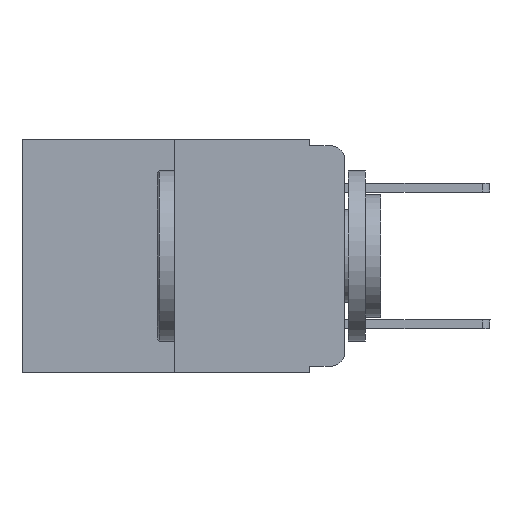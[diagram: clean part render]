
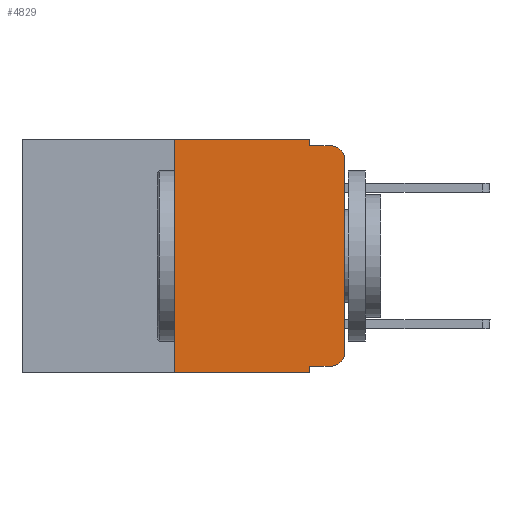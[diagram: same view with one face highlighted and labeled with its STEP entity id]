
A CAD part, left-side view. The second image highlights one B-rep face of the part: STEP entity #4829.
In plain terms, the highlighted planar face has unit normal (-1, 0, 0).
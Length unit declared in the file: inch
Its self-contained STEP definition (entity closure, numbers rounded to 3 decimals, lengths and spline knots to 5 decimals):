
#119 = CARTESIAN_POINT ( 'NONE',  ( 0., 0.25, 0. ) ) ;
#269 = DIRECTION ( 'NONE',  ( 0., 0., 1. ) ) ;
#2017 = ORIENTED_EDGE ( 'NONE', *, *, #8994, .T. ) ;
#2059 = CARTESIAN_POINT ( 'NONE',  ( 0., 0.051, 0. ) ) ;
#2314 = DIRECTION ( 'NONE',  ( 0., 0., -1. ) ) ;
#2352 = LINE ( 'NONE', #2059, #9926 ) ;
#2513 = CARTESIAN_POINT ( 'NONE',  ( 0., 0.051, 0. ) ) ;
#2537 = VECTOR ( 'NONE', #18126, 39.37008 ) ;
#2985 = ORIENTED_EDGE ( 'NONE', *, *, #7455, .T. ) ;
#3214 = VERTEX_POINT ( 'NONE', #12485 ) ;
#3493 = CARTESIAN_POINT ( 'NONE',  ( 0., 0.473, 0. ) ) ;
#3868 = ORIENTED_EDGE ( 'NONE', *, *, #16615, .T. ) ;
#4252 = CARTESIAN_POINT ( 'NONE',  ( 0., 0.051, -0.333 ) ) ;
#4829 = ADVANCED_FACE ( 'NONE', ( #7254 ), #5104, .F. ) ;
#5104 = PLANE ( 'NONE',  #19816 ) ;
#5206 = CARTESIAN_POINT ( 'NONE',  ( 0., 0.02, -0.01 ) ) ;
#5267 = CARTESIAN_POINT ( 'NONE',  ( 0., 0.051, -0.343 ) ) ;
#5402 = ORIENTED_EDGE ( 'NONE', *, *, #12630, .F. ) ;
#5836 = CIRCLE ( 'NONE', #9157, 0.02 ) ;
#5852 = ORIENTED_EDGE ( 'NONE', *, *, #18767, .F. ) ;
#6549 = EDGE_CURVE ( 'NONE', #10947, #18829, #18730, .T. ) ;
#6596 = CARTESIAN_POINT ( 'NONE',  ( 0., 0.473, 0. ) ) ;
#6755 = CARTESIAN_POINT ( 'NONE',  ( 0., 0.25, 0. ) ) ;
#6917 = VECTOR ( 'NONE', #20727, 39.37008 ) ;
#7033 = DIRECTION ( 'NONE',  ( 0., 0., -1. ) ) ;
#7208 = VERTEX_POINT ( 'NONE', #19360 ) ;
#7254 = FACE_OUTER_BOUND ( 'NONE', #12192, .T. ) ;
#7363 = LINE ( 'NONE', #6755, #19156 ) ;
#7409 = CARTESIAN_POINT ( 'NONE',  ( 0., 0., -0.03 ) ) ;
#7455 = EDGE_CURVE ( 'NONE', #20374, #13976, #18947, .T. ) ;
#7466 = ORIENTED_EDGE ( 'NONE', *, *, #17166, .T. ) ;
#7509 = CARTESIAN_POINT ( 'NONE',  ( 0., 0., 0. ) ) ;
#7764 = ORIENTED_EDGE ( 'NONE', *, *, #14862, .T. ) ;
#7814 = VERTEX_POINT ( 'NONE', #18473 ) ;
#8141 = CARTESIAN_POINT ( 'NONE',  ( 0., 0.051, 0. ) ) ;
#8751 = LINE ( 'NONE', #3493, #16274 ) ;
#8805 = CARTESIAN_POINT ( 'NONE',  ( 0., 0.02, -0.03 ) ) ;
#8957 = DIRECTION ( 'NONE',  ( 0., 0., 1. ) ) ;
#8964 = EDGE_CURVE ( 'NONE', #7208, #14667, #7363, .T. ) ;
#8994 = EDGE_CURVE ( 'NONE', #20361, #7814, #5836, .T. ) ;
#9001 = EDGE_CURVE ( 'NONE', #17385, #3214, #2352, .T. ) ;
#9157 = AXIS2_PLACEMENT_3D ( 'NONE', #10116, #10189, #7033 ) ;
#9716 = LINE ( 'NONE', #4252, #6917 ) ;
#9736 = VECTOR ( 'NONE', #13779, 39.37008 ) ;
#9838 = ORIENTED_EDGE ( 'NONE', *, *, #8964, .F. ) ;
#9926 = VECTOR ( 'NONE', #11877, 39.37008 ) ;
#10116 = CARTESIAN_POINT ( 'NONE',  ( 0., 0.02, -0.313 ) ) ;
#10189 = DIRECTION ( 'NONE',  ( -1., 0., 0. ) ) ;
#10475 = VECTOR ( 'NONE', #14422, 39.37008 ) ;
#10500 = CARTESIAN_POINT ( 'NONE',  ( 0., 0.02, -0.333 ) ) ;
#10947 = VERTEX_POINT ( 'NONE', #12155 ) ;
#11160 = ORIENTED_EDGE ( 'NONE', *, *, #6549, .F. ) ;
#11381 = DIRECTION ( 'NONE',  ( 1., 0., 0. ) ) ;
#11719 = DIRECTION ( 'NONE',  ( -1., 0., 0. ) ) ;
#11877 = DIRECTION ( 'NONE',  ( 0., 0., -1. ) ) ;
#12155 = CARTESIAN_POINT ( 'NONE',  ( 0., 0.051, -0.333 ) ) ;
#12192 = EDGE_LOOP ( 'NONE', ( #7764, #2985, #5852, #12451, #5402, #9838, #3868, #11160, #7466, #2017 ) ) ;
#12451 = ORIENTED_EDGE ( 'NONE', *, *, #9001, .F. ) ;
#12485 = CARTESIAN_POINT ( 'NONE',  ( 0., 0.051, -0.01 ) ) ;
#12630 = EDGE_CURVE ( 'NONE', #14667, #17385, #8751, .T. ) ;
#13048 = VECTOR ( 'NONE', #8957, 39.37008 ) ;
#13705 = LINE ( 'NONE', #17090, #10475 ) ;
#13779 = DIRECTION ( 'NONE',  ( 0., 0., -1. ) ) ;
#13974 = AXIS2_PLACEMENT_3D ( 'NONE', #8805, #11719, #2314 ) ;
#13976 = VERTEX_POINT ( 'NONE', #5206 ) ;
#14363 = LINE ( 'NONE', #14859, #2537 ) ;
#14422 = DIRECTION ( 'NONE',  ( 0., -1., 0. ) ) ;
#14635 = DIRECTION ( 'NONE',  ( 0., -1., 0. ) ) ;
#14667 = VERTEX_POINT ( 'NONE', #119 ) ;
#14859 = CARTESIAN_POINT ( 'NONE',  ( 0., 0.051, -0.01 ) ) ;
#14862 = EDGE_CURVE ( 'NONE', #7814, #20374, #19787, .T. ) ;
#16274 = VECTOR ( 'NONE', #14635, 39.37008 ) ;
#16615 = EDGE_CURVE ( 'NONE', #7208, #18829, #13705, .T. ) ;
#17090 = CARTESIAN_POINT ( 'NONE',  ( 0., 0.473, -0.343 ) ) ;
#17166 = EDGE_CURVE ( 'NONE', #10947, #20361, #9716, .T. ) ;
#17385 = VERTEX_POINT ( 'NONE', #8141 ) ;
#18126 = DIRECTION ( 'NONE',  ( 0., -1., 0. ) ) ;
#18473 = CARTESIAN_POINT ( 'NONE',  ( 0., 0., -0.313 ) ) ;
#18730 = LINE ( 'NONE', #2513, #9736 ) ;
#18767 = EDGE_CURVE ( 'NONE', #3214, #13976, #14363, .T. ) ;
#18829 = VERTEX_POINT ( 'NONE', #5267 ) ;
#18947 = CIRCLE ( 'NONE', #13974, 0.02 ) ;
#19156 = VECTOR ( 'NONE', #269, 39.37008 ) ;
#19237 = DIRECTION ( 'NONE',  ( 0., 0., -1. ) ) ;
#19360 = CARTESIAN_POINT ( 'NONE',  ( 0., 0.25, -0.343 ) ) ;
#19787 = LINE ( 'NONE', #7509, #13048 ) ;
#19816 = AXIS2_PLACEMENT_3D ( 'NONE', #6596, #11381, #19237 ) ;
#20361 = VERTEX_POINT ( 'NONE', #10500 ) ;
#20374 = VERTEX_POINT ( 'NONE', #7409 ) ;
#20727 = DIRECTION ( 'NONE',  ( 0., -1., 0. ) ) ;
